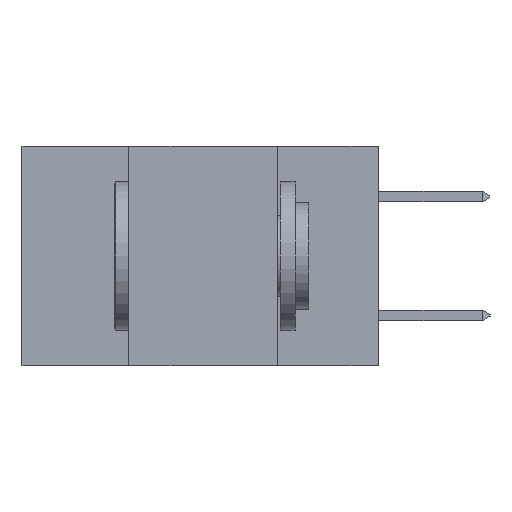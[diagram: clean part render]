
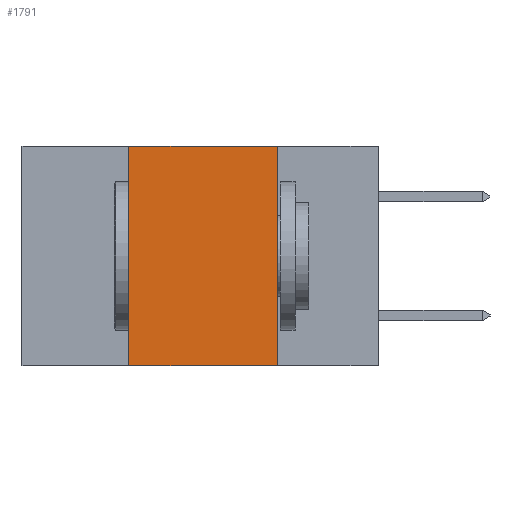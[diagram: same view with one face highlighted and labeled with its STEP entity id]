
A CAD part, left-side view. The second image highlights one B-rep face of the part: STEP entity #1791.
In plain terms, the highlighted planar face has unit normal (-1, 0, 0).
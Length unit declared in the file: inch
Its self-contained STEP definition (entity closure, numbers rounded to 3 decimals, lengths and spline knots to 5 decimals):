
#221 = LINE ( 'NONE', #13164, #15432 ) ;
#228 = ORIENTED_EDGE ( 'NONE', *, *, #21686, .F. ) ;
#400 = VERTEX_POINT ( 'NONE', #7904 ) ;
#575 = DIRECTION ( 'NONE',  ( 0., 0., -1. ) ) ;
#1526 = DIRECTION ( 'NONE',  ( 0., 0., 1. ) ) ;
#1644 = VECTOR ( 'NONE', #16849, 39.37008 ) ;
#1791 = ADVANCED_FACE ( 'NONE', ( #22651 ), #25237, .F. ) ;
#2380 = EDGE_CURVE ( 'NONE', #23790, #18871, #19543, .T. ) ;
#4176 = ORIENTED_EDGE ( 'NONE', *, *, #13542, .F. ) ;
#7904 = CARTESIAN_POINT ( 'NONE',  ( 0., 0.42, 0. ) ) ;
#8069 = CARTESIAN_POINT ( 'NONE',  ( 0., 0.17, -0.37 ) ) ;
#8119 = AXIS2_PLACEMENT_3D ( 'NONE', #19588, #17347, #575 ) ;
#9083 = VECTOR ( 'NONE', #1526, 39.37008 ) ;
#13164 = CARTESIAN_POINT ( 'NONE',  ( 0., 0.6, -0.37 ) ) ;
#13542 = EDGE_CURVE ( 'NONE', #22721, #400, #25815, .T. ) ;
#13633 = DIRECTION ( 'NONE',  ( 0., 0., -1. ) ) ;
#14911 = CARTESIAN_POINT ( 'NONE',  ( 0., 0.42, -0.37 ) ) ;
#14917 = CARTESIAN_POINT ( 'NONE',  ( 0., 0.17, -0.37 ) ) ;
#15432 = VECTOR ( 'NONE', #21318, 39.37008 ) ;
#16849 = DIRECTION ( 'NONE',  ( 0., -1., 0. ) ) ;
#17031 = ORIENTED_EDGE ( 'NONE', *, *, #2380, .F. ) ;
#17347 = DIRECTION ( 'NONE',  ( 1., 0., 0. ) ) ;
#18871 = VERTEX_POINT ( 'NONE', #8069 ) ;
#18912 = VECTOR ( 'NONE', #13633, 39.37008 ) ;
#18969 = ORIENTED_EDGE ( 'NONE', *, *, #23493, .T. ) ;
#19543 = LINE ( 'NONE', #14917, #18912 ) ;
#19588 = CARTESIAN_POINT ( 'NONE',  ( 0., 0.6, 0. ) ) ;
#20467 = CARTESIAN_POINT ( 'NONE',  ( 0., 0.17, 0. ) ) ;
#21318 = DIRECTION ( 'NONE',  ( 0., -1., 0. ) ) ;
#21686 = EDGE_CURVE ( 'NONE', #400, #23790, #23358, .T. ) ;
#21756 = EDGE_LOOP ( 'NONE', ( #17031, #228, #4176, #18969 ) ) ;
#22651 = FACE_OUTER_BOUND ( 'NONE', #21756, .T. ) ;
#22721 = VERTEX_POINT ( 'NONE', #14911 ) ;
#22768 = CARTESIAN_POINT ( 'NONE',  ( 0., 0.6, 0. ) ) ;
#23358 = LINE ( 'NONE', #22768, #1644 ) ;
#23493 = EDGE_CURVE ( 'NONE', #22721, #18871, #221, .T. ) ;
#23790 = VERTEX_POINT ( 'NONE', #20467 ) ;
#25237 = PLANE ( 'NONE',  #8119 ) ;
#25815 = LINE ( 'NONE', #25878, #9083 ) ;
#25878 = CARTESIAN_POINT ( 'NONE',  ( 0., 0.42, -0.37 ) ) ;
